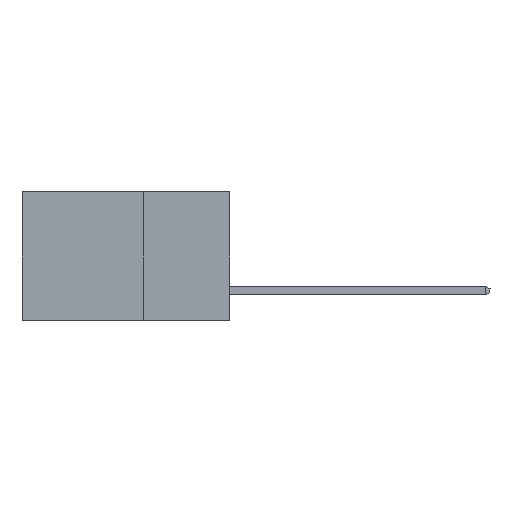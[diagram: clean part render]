
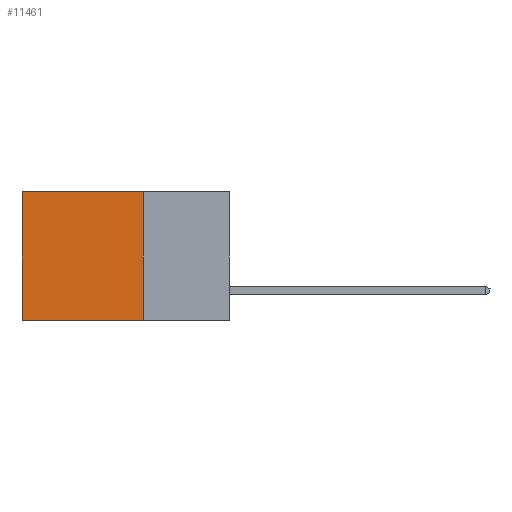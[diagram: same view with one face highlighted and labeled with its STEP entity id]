
A CAD part, left-side view. The second image highlights one B-rep face of the part: STEP entity #11461.
In plain terms, the highlighted planar face has unit normal (-1, 0, 0).
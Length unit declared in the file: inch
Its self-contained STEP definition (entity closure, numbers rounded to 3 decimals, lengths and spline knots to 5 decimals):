
#242 = FACE_OUTER_BOUND ( 'NONE', #6457, .T. ) ;
#819 = LINE ( 'NONE', #12230, #1419 ) ;
#953 = LINE ( 'NONE', #4864, #8000 ) ;
#1064 = ORIENTED_EDGE ( 'NONE', *, *, #10505, .T. ) ;
#1419 = VECTOR ( 'NONE', #13094, 39.37008 ) ;
#1578 = CARTESIAN_POINT ( 'NONE',  ( 0.2615, 0.25, -0.37 ) ) ;
#1943 = DIRECTION ( 'NONE',  ( 0., 1., 0. ) ) ;
#2122 = EDGE_CURVE ( 'NONE', #3649, #13120, #2565, .T. ) ;
#2486 = DIRECTION ( 'NONE',  ( 1., 0., 0. ) ) ;
#2511 = EDGE_CURVE ( 'NONE', #5187, #3983, #4914, .T. ) ;
#2565 = LINE ( 'NONE', #1578, #9773 ) ;
#3073 = CARTESIAN_POINT ( 'NONE',  ( 0.2615, 0.6, -0.37 ) ) ;
#3649 = VERTEX_POINT ( 'NONE', #10287 ) ;
#3983 = VERTEX_POINT ( 'NONE', #3073 ) ;
#4146 = ORIENTED_EDGE ( 'NONE', *, *, #10430, .F. ) ;
#4413 = DIRECTION ( 'NONE',  ( 0., 0., -1. ) ) ;
#4864 = CARTESIAN_POINT ( 'NONE',  ( 0.2615, 0.25, 0. ) ) ;
#4914 = LINE ( 'NONE', #7796, #8911 ) ;
#4993 = CARTESIAN_POINT ( 'NONE',  ( 0.2615, 0.6, 0. ) ) ;
#5187 = VERTEX_POINT ( 'NONE', #4993 ) ;
#5408 = PLANE ( 'NONE',  #10817 ) ;
#6457 = EDGE_LOOP ( 'NONE', ( #12004, #4146, #10932, #1064 ) ) ;
#6615 = CARTESIAN_POINT ( 'NONE',  ( 0.2615, 0.25, -0.37 ) ) ;
#7796 = CARTESIAN_POINT ( 'NONE',  ( 0.2615, 0.6, -0.37 ) ) ;
#8000 = VECTOR ( 'NONE', #1943, 39.37008 ) ;
#8911 = VECTOR ( 'NONE', #8915, 39.37008 ) ;
#8915 = DIRECTION ( 'NONE',  ( 0., 0., -1. ) ) ;
#9760 = DIRECTION ( 'NONE',  ( 0., 0., -1. ) ) ;
#9773 = VECTOR ( 'NONE', #9760, 39.37008 ) ;
#10287 = CARTESIAN_POINT ( 'NONE',  ( 0.2615, 0.25, 0. ) ) ;
#10430 = EDGE_CURVE ( 'NONE', #13120, #3983, #819, .T. ) ;
#10505 = EDGE_CURVE ( 'NONE', #3649, #5187, #953, .T. ) ;
#10625 = CARTESIAN_POINT ( 'NONE',  ( 0.2615, 0.25, -0.37 ) ) ;
#10817 = AXIS2_PLACEMENT_3D ( 'NONE', #10625, #2486, #4413 ) ;
#10932 = ORIENTED_EDGE ( 'NONE', *, *, #2122, .F. ) ;
#11461 = ADVANCED_FACE ( 'NONE', ( #242 ), #5408, .F. ) ;
#12004 = ORIENTED_EDGE ( 'NONE', *, *, #2511, .T. ) ;
#12230 = CARTESIAN_POINT ( 'NONE',  ( 0.2615, 0.25, -0.37 ) ) ;
#13094 = DIRECTION ( 'NONE',  ( 0., 1., 0. ) ) ;
#13120 = VERTEX_POINT ( 'NONE', #6615 ) ;
